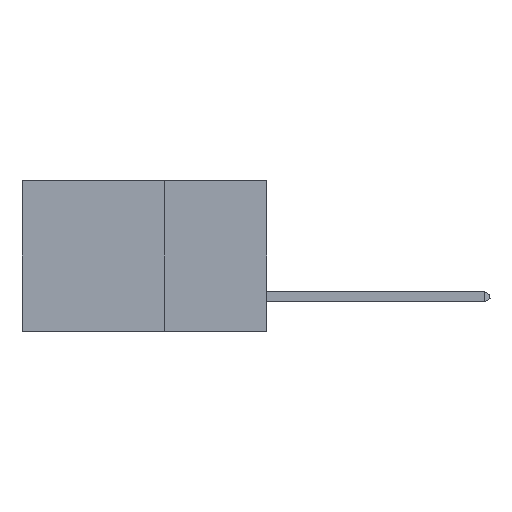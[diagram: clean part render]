
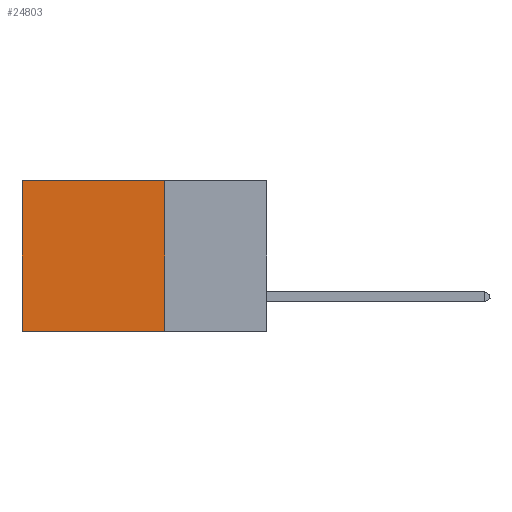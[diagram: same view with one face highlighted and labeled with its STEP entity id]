
A CAD part, left-side view. The second image highlights one B-rep face of the part: STEP entity #24803.
In plain terms, the highlighted planar face has unit normal (-1, 0, 0).
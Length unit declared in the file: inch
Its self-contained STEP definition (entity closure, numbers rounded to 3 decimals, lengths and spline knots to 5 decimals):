
#1410 = ORIENTED_EDGE ( 'NONE', *, *, #22426, .T. ) ;
#2899 = ORIENTED_EDGE ( 'NONE', *, *, #34179, .F. ) ;
#5404 = CARTESIAN_POINT ( 'NONE',  ( 0.2875, 0.25, -0.37 ) ) ;
#6894 = VECTOR ( 'NONE', #21325, 39.37008 ) ;
#7269 = CARTESIAN_POINT ( 'NONE',  ( 0.2875, 0.25, 0. ) ) ;
#8999 = CARTESIAN_POINT ( 'NONE',  ( 0.2875, 0.6, -0.37 ) ) ;
#11503 = FACE_OUTER_BOUND ( 'NONE', #22839, .T. ) ;
#12235 = PLANE ( 'NONE',  #20937 ) ;
#12958 = ORIENTED_EDGE ( 'NONE', *, *, #38367, .F. ) ;
#13168 = LINE ( 'NONE', #35280, #30282 ) ;
#13397 = DIRECTION ( 'NONE',  ( 0., 0., -1. ) ) ;
#16626 = CARTESIAN_POINT ( 'NONE',  ( 0.2875, 0.6, 0. ) ) ;
#17768 = CARTESIAN_POINT ( 'NONE',  ( 0.2875, 0.6, 0. ) ) ;
#18511 = DIRECTION ( 'NONE',  ( 1., 0., 0. ) ) ;
#20937 = AXIS2_PLACEMENT_3D ( 'NONE', #37135, #18511, #21676 ) ;
#21325 = DIRECTION ( 'NONE',  ( 0., 1., 0. ) ) ;
#21516 = CARTESIAN_POINT ( 'NONE',  ( 0.2875, 0.25, -0.37 ) ) ;
#21650 = EDGE_CURVE ( 'NONE', #33278, #22852, #30787, .T. ) ;
#21676 = DIRECTION ( 'NONE',  ( 0., 0., -1. ) ) ;
#22426 = EDGE_CURVE ( 'NONE', #22481, #33278, #26826, .T. ) ;
#22481 = VERTEX_POINT ( 'NONE', #26331 ) ;
#22839 = EDGE_LOOP ( 'NONE', ( #32607, #2899, #12958, #1410 ) ) ;
#22852 = VERTEX_POINT ( 'NONE', #8999 ) ;
#22942 = DIRECTION ( 'NONE',  ( 0., 0., -1. ) ) ;
#24803 = ADVANCED_FACE ( 'NONE', ( #11503 ), #12235, .F. ) ;
#26331 = CARTESIAN_POINT ( 'NONE',  ( 0.2875, 0.25, 0. ) ) ;
#26826 = LINE ( 'NONE', #7269, #31662 ) ;
#30282 = VECTOR ( 'NONE', #13397, 39.37008 ) ;
#30332 = VECTOR ( 'NONE', #22942, 39.37008 ) ;
#30787 = LINE ( 'NONE', #16626, #30332 ) ;
#31662 = VECTOR ( 'NONE', #31882, 39.37008 ) ;
#31882 = DIRECTION ( 'NONE',  ( 0., 1., 0. ) ) ;
#32607 = ORIENTED_EDGE ( 'NONE', *, *, #21650, .T. ) ;
#33278 = VERTEX_POINT ( 'NONE', #17768 ) ;
#34179 = EDGE_CURVE ( 'NONE', #39481, #22852, #35577, .T. ) ;
#35280 = CARTESIAN_POINT ( 'NONE',  ( 0.2875, 0.25, 0. ) ) ;
#35577 = LINE ( 'NONE', #5404, #6894 ) ;
#37135 = CARTESIAN_POINT ( 'NONE',  ( 0.2875, 0.25, 0. ) ) ;
#38367 = EDGE_CURVE ( 'NONE', #22481, #39481, #13168, .T. ) ;
#39481 = VERTEX_POINT ( 'NONE', #21516 ) ;
